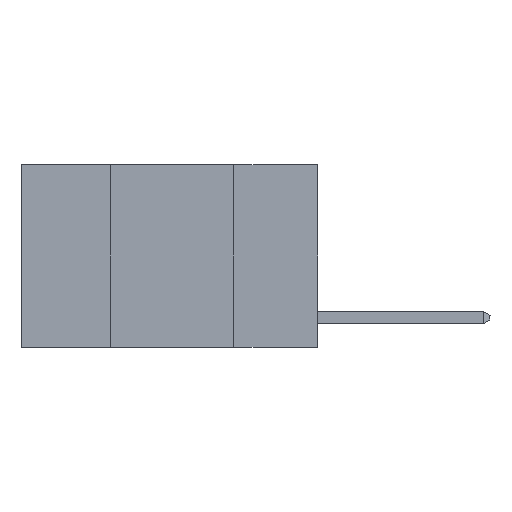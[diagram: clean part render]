
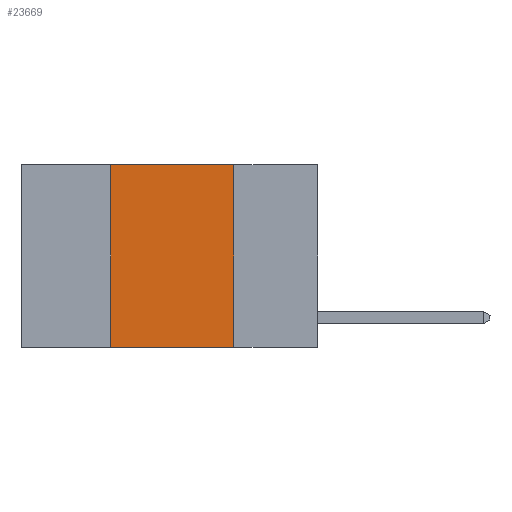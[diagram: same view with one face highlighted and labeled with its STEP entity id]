
A CAD part, left-side view. The second image highlights one B-rep face of the part: STEP entity #23669.
In plain terms, the highlighted planar face has unit normal (-1, 0, 0).
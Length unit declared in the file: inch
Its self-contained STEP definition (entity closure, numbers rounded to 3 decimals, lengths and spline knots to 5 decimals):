
#344 = EDGE_CURVE ( 'NONE', #4427, #11839, #15911, .T. ) ;
#618 = DIRECTION ( 'NONE',  ( 0., 0., 1. ) ) ;
#1290 = LINE ( 'NONE', #5465, #15662 ) ;
#1916 = ORIENTED_EDGE ( 'NONE', *, *, #6983, .T. ) ;
#2052 = VERTEX_POINT ( 'NONE', #20375 ) ;
#2203 = CARTESIAN_POINT ( 'NONE',  ( 0., 0.42, 0. ) ) ;
#2402 = DIRECTION ( 'NONE',  ( 0., -1., 0. ) ) ;
#3678 = ORIENTED_EDGE ( 'NONE', *, *, #21826, .F. ) ;
#4427 = VERTEX_POINT ( 'NONE', #6047 ) ;
#4728 = FACE_OUTER_BOUND ( 'NONE', #21577, .T. ) ;
#5130 = DIRECTION ( 'NONE',  ( 0., 0., -1. ) ) ;
#5465 = CARTESIAN_POINT ( 'NONE',  ( 0., 0.17, 0. ) ) ;
#6047 = CARTESIAN_POINT ( 'NONE',  ( 0., 0.42, -0.37 ) ) ;
#6096 = CARTESIAN_POINT ( 'NONE',  ( 0., 0.6, -0.37 ) ) ;
#6803 = ORIENTED_EDGE ( 'NONE', *, *, #6839, .F. ) ;
#6839 = EDGE_CURVE ( 'NONE', #21146, #2052, #1290, .T. ) ;
#6983 = EDGE_CURVE ( 'NONE', #4427, #2052, #11470, .T. ) ;
#7591 = DIRECTION ( 'NONE',  ( 0., -1., 0. ) ) ;
#7749 = VECTOR ( 'NONE', #618, 39.37008 ) ;
#7813 = CARTESIAN_POINT ( 'NONE',  ( 0., 0.17, 0. ) ) ;
#9026 = DIRECTION ( 'NONE',  ( 1., 0., 0. ) ) ;
#11470 = LINE ( 'NONE', #6096, #20907 ) ;
#11839 = VERTEX_POINT ( 'NONE', #2203 ) ;
#12439 = PLANE ( 'NONE',  #19419 ) ;
#14703 = CARTESIAN_POINT ( 'NONE',  ( 0., 0.6, 0. ) ) ;
#15662 = VECTOR ( 'NONE', #17200, 39.37008 ) ;
#15911 = LINE ( 'NONE', #21715, #7749 ) ;
#16562 = LINE ( 'NONE', #14703, #20964 ) ;
#16611 = CARTESIAN_POINT ( 'NONE',  ( 0., 0.6, 0. ) ) ;
#16626 = ORIENTED_EDGE ( 'NONE', *, *, #344, .F. ) ;
#17200 = DIRECTION ( 'NONE',  ( 0., 0., -1. ) ) ;
#19419 = AXIS2_PLACEMENT_3D ( 'NONE', #16611, #9026, #5130 ) ;
#20375 = CARTESIAN_POINT ( 'NONE',  ( 0., 0.17, -0.37 ) ) ;
#20907 = VECTOR ( 'NONE', #2402, 39.37008 ) ;
#20964 = VECTOR ( 'NONE', #7591, 39.37008 ) ;
#21146 = VERTEX_POINT ( 'NONE', #7813 ) ;
#21577 = EDGE_LOOP ( 'NONE', ( #6803, #3678, #16626, #1916 ) ) ;
#21715 = CARTESIAN_POINT ( 'NONE',  ( 0., 0.42, 0. ) ) ;
#21826 = EDGE_CURVE ( 'NONE', #11839, #21146, #16562, .T. ) ;
#23669 = ADVANCED_FACE ( 'NONE', ( #4728 ), #12439, .F. ) ;
